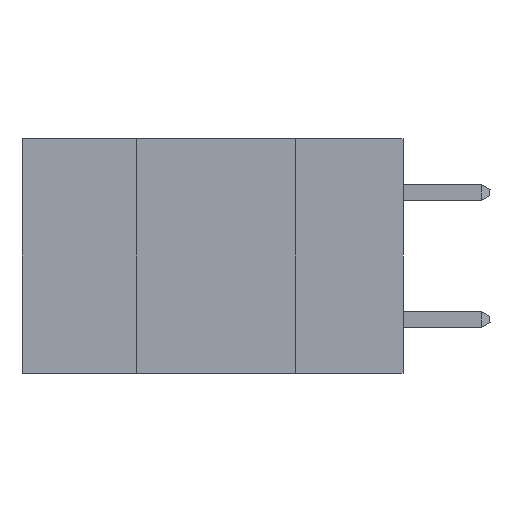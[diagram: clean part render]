
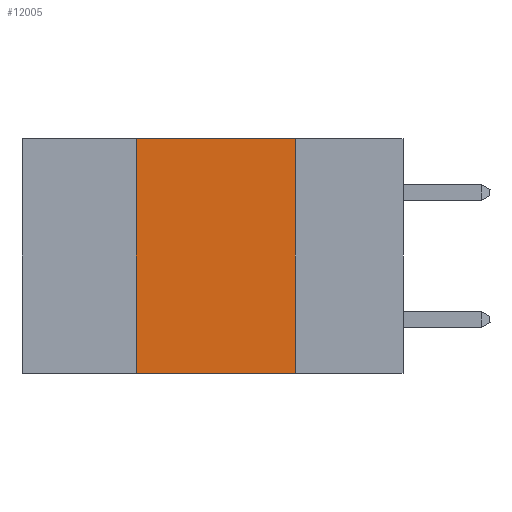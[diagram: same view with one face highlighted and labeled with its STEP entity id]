
A CAD part, left-side view. The second image highlights one B-rep face of the part: STEP entity #12005.
In plain terms, the highlighted planar face has unit normal (-1, 0, 0).
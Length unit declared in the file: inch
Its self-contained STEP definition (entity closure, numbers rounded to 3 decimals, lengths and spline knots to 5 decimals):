
#809 = VERTEX_POINT ( 'NONE', #13909 ) ;
#1106 = CARTESIAN_POINT ( 'NONE',  ( 0., 0.6, 0. ) ) ;
#1328 = DIRECTION ( 'NONE',  ( 0., 0., -1. ) ) ;
#3041 = LINE ( 'NONE', #1106, #7243 ) ;
#4734 = CARTESIAN_POINT ( 'NONE',  ( 0., 0.42, 0. ) ) ;
#5300 = VECTOR ( 'NONE', #34308, 39.37008 ) ;
#7110 = DIRECTION ( 'NONE',  ( 0., 0., -1. ) ) ;
#7238 = VECTOR ( 'NONE', #7110, 39.37008 ) ;
#7243 = VECTOR ( 'NONE', #22674, 39.37008 ) ;
#9116 = CARTESIAN_POINT ( 'NONE',  ( 0., 0.42, 0. ) ) ;
#9942 = CARTESIAN_POINT ( 'NONE',  ( 0., 0.6, 0. ) ) ;
#12005 = ADVANCED_FACE ( 'NONE', ( #25242 ), #15033, .F. ) ;
#13909 = CARTESIAN_POINT ( 'NONE',  ( 0., 0.42, -0.37 ) ) ;
#15033 = PLANE ( 'NONE',  #20913 ) ;
#15451 = LINE ( 'NONE', #31224, #5300 ) ;
#16294 = VERTEX_POINT ( 'NONE', #4734 ) ;
#16549 = LINE ( 'NONE', #34107, #7238 ) ;
#18541 = EDGE_LOOP ( 'NONE', ( #29164, #24299, #33724, #25727 ) ) ;
#20913 = AXIS2_PLACEMENT_3D ( 'NONE', #9942, #28891, #1328 ) ;
#21334 = EDGE_CURVE ( 'NONE', #809, #31234, #15451, .T. ) ;
#21727 = CARTESIAN_POINT ( 'NONE',  ( 0., 0.17, 0. ) ) ;
#22674 = DIRECTION ( 'NONE',  ( 0., -1., 0. ) ) ;
#24299 = ORIENTED_EDGE ( 'NONE', *, *, #25878, .F. ) ;
#25242 = FACE_OUTER_BOUND ( 'NONE', #18541, .T. ) ;
#25669 = VERTEX_POINT ( 'NONE', #21727 ) ;
#25727 = ORIENTED_EDGE ( 'NONE', *, *, #21334, .T. ) ;
#25878 = EDGE_CURVE ( 'NONE', #16294, #25669, #3041, .T. ) ;
#26569 = LINE ( 'NONE', #9116, #32926 ) ;
#27540 = EDGE_CURVE ( 'NONE', #809, #16294, #26569, .T. ) ;
#28891 = DIRECTION ( 'NONE',  ( 1., 0., 0. ) ) ;
#29164 = ORIENTED_EDGE ( 'NONE', *, *, #31050, .F. ) ;
#31050 = EDGE_CURVE ( 'NONE', #25669, #31234, #16549, .T. ) ;
#31224 = CARTESIAN_POINT ( 'NONE',  ( 0., 0.6, -0.37 ) ) ;
#31234 = VERTEX_POINT ( 'NONE', #34235 ) ;
#32926 = VECTOR ( 'NONE', #33974, 39.37008 ) ;
#33724 = ORIENTED_EDGE ( 'NONE', *, *, #27540, .F. ) ;
#33974 = DIRECTION ( 'NONE',  ( 0., 0., 1. ) ) ;
#34107 = CARTESIAN_POINT ( 'NONE',  ( 0., 0.17, 0. ) ) ;
#34235 = CARTESIAN_POINT ( 'NONE',  ( 0., 0.17, -0.37 ) ) ;
#34308 = DIRECTION ( 'NONE',  ( 0., -1., 0. ) ) ;
